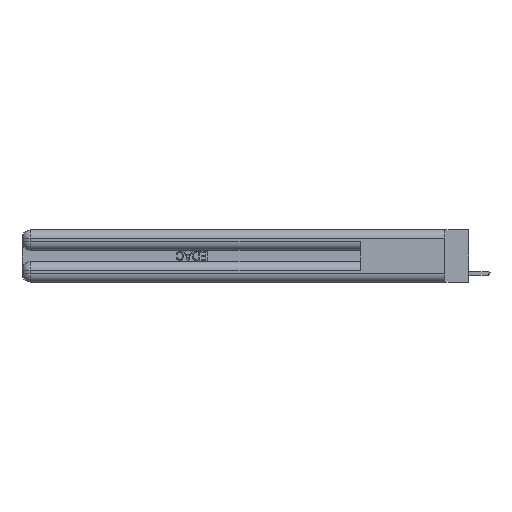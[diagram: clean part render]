
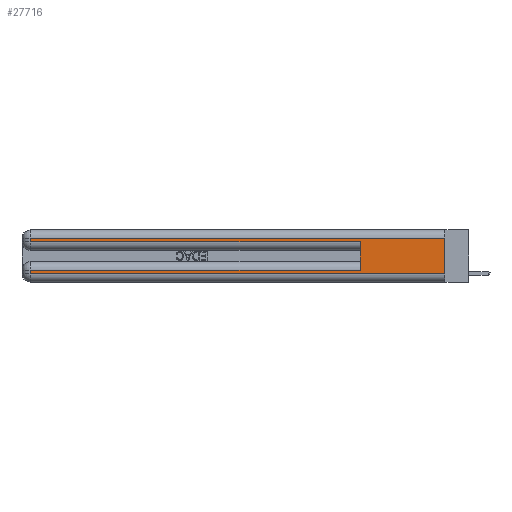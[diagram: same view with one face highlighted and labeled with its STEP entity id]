
A CAD part, left-side view. The second image highlights one B-rep face of the part: STEP entity #27716.
In plain terms, the highlighted planar face has unit normal (-1, 0, 0).
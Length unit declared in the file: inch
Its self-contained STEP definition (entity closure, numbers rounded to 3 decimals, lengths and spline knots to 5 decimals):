
#879 = ORIENTED_EDGE ( 'NONE', *, *, #6931, .T. ) ;
#1299 = VERTEX_POINT ( 'NONE', #8098 ) ;
#1821 = VECTOR ( 'NONE', #19691, 39.37008 ) ;
#2665 = CARTESIAN_POINT ( 'NONE',  ( 0., 2.94, 0.37 ) ) ;
#2706 = EDGE_CURVE ( 'NONE', #28455, #21421, #13916, .T. ) ;
#2883 = CARTESIAN_POINT ( 'NONE',  ( 0., 2.94, 0.085 ) ) ;
#3244 = AXIS2_PLACEMENT_3D ( 'NONE', #26540, #14114, #24095 ) ;
#3841 = DIRECTION ( 'NONE',  ( 0., 0., 1. ) ) ;
#4134 = CARTESIAN_POINT ( 'NONE',  ( 0., 2.94, 0.37 ) ) ;
#5106 = LINE ( 'NONE', #2665, #13583 ) ;
#6621 = CARTESIAN_POINT ( 'NONE',  ( 0., 2.94, 0.285 ) ) ;
#6624 = CARTESIAN_POINT ( 'NONE',  ( 0., 2.94, 0.06 ) ) ;
#6790 = CARTESIAN_POINT ( 'NONE',  ( 0., 0., 0.31 ) ) ;
#6931 = EDGE_CURVE ( 'NONE', #1299, #28455, #5106, .T. ) ;
#6941 = LINE ( 'NONE', #24298, #8528 ) ;
#7275 = LINE ( 'NONE', #9398, #14009 ) ;
#7303 = CARTESIAN_POINT ( 'NONE',  ( 0., 0., 0.31 ) ) ;
#7615 = EDGE_CURVE ( 'NONE', #13243, #8078, #29578, .T. ) ;
#7784 = DIRECTION ( 'NONE',  ( 0., 1., 0. ) ) ;
#7898 = EDGE_LOOP ( 'NONE', ( #20068, #21207, #879, #18903, #27942, #17681, #23862, #21098 ) ) ;
#8078 = VERTEX_POINT ( 'NONE', #12648 ) ;
#8098 = CARTESIAN_POINT ( 'NONE',  ( 0., 2.94, 0.31 ) ) ;
#8429 = VECTOR ( 'NONE', #7784, 39.37008 ) ;
#8528 = VECTOR ( 'NONE', #3841, 39.37008 ) ;
#9044 = LINE ( 'NONE', #4134, #1821 ) ;
#9382 = EDGE_CURVE ( 'NONE', #14614, #8078, #24966, .T. ) ;
#9398 = CARTESIAN_POINT ( 'NONE',  ( 0., 0., 0.085 ) ) ;
#11457 = CARTESIAN_POINT ( 'NONE',  ( 0., 0., 0.285 ) ) ;
#11497 = FACE_OUTER_BOUND ( 'NONE', #7898, .T. ) ;
#12645 = DIRECTION ( 'NONE',  ( 0., 0., -1. ) ) ;
#12648 = CARTESIAN_POINT ( 'NONE',  ( 0., 0., 0.06 ) ) ;
#13243 = VERTEX_POINT ( 'NONE', #6624 ) ;
#13583 = VECTOR ( 'NONE', #12645, 39.37008 ) ;
#13916 = LINE ( 'NONE', #11457, #21602 ) ;
#14009 = VECTOR ( 'NONE', #32298, 39.37008 ) ;
#14114 = DIRECTION ( 'NONE',  ( 1., 0., 0. ) ) ;
#14614 = VERTEX_POINT ( 'NONE', #6790 ) ;
#16194 = EDGE_CURVE ( 'NONE', #28155, #13243, #9044, .T. ) ;
#16828 = DIRECTION ( 'NONE',  ( 0., -1., 0. ) ) ;
#17681 = ORIENTED_EDGE ( 'NONE', *, *, #20229, .T. ) ;
#17802 = VERTEX_POINT ( 'NONE', #24563 ) ;
#18903 = ORIENTED_EDGE ( 'NONE', *, *, #2706, .T. ) ;
#19691 = DIRECTION ( 'NONE',  ( 0., 0., -1. ) ) ;
#20068 = ORIENTED_EDGE ( 'NONE', *, *, #9382, .F. ) ;
#20229 = EDGE_CURVE ( 'NONE', #17802, #28155, #7275, .T. ) ;
#21098 = ORIENTED_EDGE ( 'NONE', *, *, #7615, .T. ) ;
#21207 = ORIENTED_EDGE ( 'NONE', *, *, #26921, .T. ) ;
#21261 = CARTESIAN_POINT ( 'NONE',  ( 0., 0.6, 0.285 ) ) ;
#21421 = VERTEX_POINT ( 'NONE', #21261 ) ;
#21602 = VECTOR ( 'NONE', #21607, 39.37008 ) ;
#21607 = DIRECTION ( 'NONE',  ( 0., -1., 0. ) ) ;
#21721 = VECTOR ( 'NONE', #16828, 39.37008 ) ;
#23862 = ORIENTED_EDGE ( 'NONE', *, *, #16194, .T. ) ;
#24095 = DIRECTION ( 'NONE',  ( 0., 0., -1. ) ) ;
#24298 = CARTESIAN_POINT ( 'NONE',  ( 0., 0.6, 0.145 ) ) ;
#24447 = VECTOR ( 'NONE', #32323, 39.37008 ) ;
#24563 = CARTESIAN_POINT ( 'NONE',  ( 0., 0.6, 0.085 ) ) ;
#24966 = LINE ( 'NONE', #30346, #24447 ) ;
#26540 = CARTESIAN_POINT ( 'NONE',  ( 0., 0., 0.37 ) ) ;
#26921 = EDGE_CURVE ( 'NONE', #14614, #1299, #30034, .T. ) ;
#27716 = ADVANCED_FACE ( 'NONE', ( #11497 ), #31439, .F. ) ;
#27942 = ORIENTED_EDGE ( 'NONE', *, *, #28484, .F. ) ;
#28155 = VERTEX_POINT ( 'NONE', #2883 ) ;
#28455 = VERTEX_POINT ( 'NONE', #6621 ) ;
#28484 = EDGE_CURVE ( 'NONE', #17802, #21421, #6941, .T. ) ;
#29578 = LINE ( 'NONE', #32025, #21721 ) ;
#30034 = LINE ( 'NONE', #7303, #8429 ) ;
#30346 = CARTESIAN_POINT ( 'NONE',  ( 0., 0., 0.37 ) ) ;
#31439 = PLANE ( 'NONE',  #3244 ) ;
#32025 = CARTESIAN_POINT ( 'NONE',  ( 0., 0., 0.06 ) ) ;
#32298 = DIRECTION ( 'NONE',  ( 0., 1., 0. ) ) ;
#32323 = DIRECTION ( 'NONE',  ( 0., 0., -1. ) ) ;
